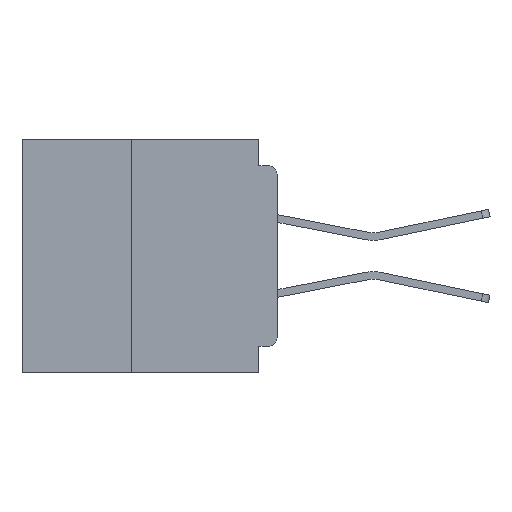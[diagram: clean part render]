
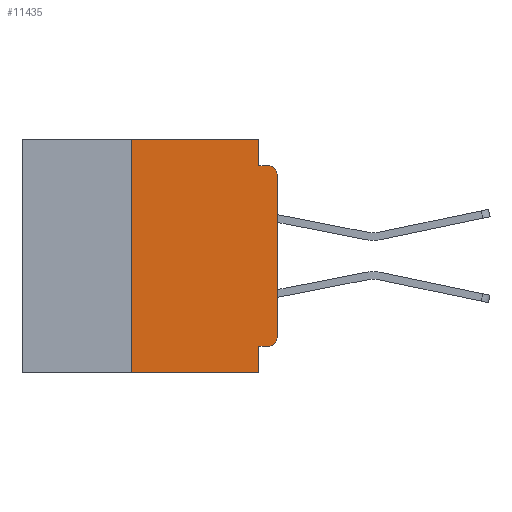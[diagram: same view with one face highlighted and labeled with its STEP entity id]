
A CAD part, left-side view. The second image highlights one B-rep face of the part: STEP entity #11435.
In plain terms, the highlighted planar face has unit normal (-1, 0, 0).
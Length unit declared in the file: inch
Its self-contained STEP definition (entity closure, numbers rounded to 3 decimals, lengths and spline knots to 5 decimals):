
#1499 = CARTESIAN_POINT ( 'NONE',  ( 0., 0.015, -0.34 ) ) ;
#1904 = CARTESIAN_POINT ( 'NONE',  ( 0., 0.437, 0. ) ) ;
#1909 = DIRECTION ( 'NONE',  ( 0., 0., -1. ) ) ;
#2004 = AXIS2_PLACEMENT_3D ( 'NONE', #1904, #37507, #13945 ) ;
#3183 = EDGE_CURVE ( 'NONE', #51028, #47397, #34733, .T. ) ;
#3277 = CARTESIAN_POINT ( 'NONE',  ( 0., 0., -0.34 ) ) ;
#4523 = DIRECTION ( 'NONE',  ( 0., -1., 0. ) ) ;
#4692 = EDGE_CURVE ( 'NONE', #48364, #48477, #16767, .T. ) ;
#5548 = DIRECTION ( 'NONE',  ( 0., 0., -1. ) ) ;
#5969 = PLANE ( 'NONE',  #2004 ) ;
#6402 = CARTESIAN_POINT ( 'NONE',  ( 0., 0.437, -0.4 ) ) ;
#7161 = VECTOR ( 'NONE', #17415, 39.37008 ) ;
#11061 = CARTESIAN_POINT ( 'NONE',  ( 0., 0.015, -0.355 ) ) ;
#11435 = ADVANCED_FACE ( 'NONE', ( #44710 ), #5969, .F. ) ;
#11974 = CARTESIAN_POINT ( 'NONE',  ( 0., 0.015, -0.045 ) ) ;
#12048 = LINE ( 'NONE', #24384, #31739 ) ;
#13144 = VECTOR ( 'NONE', #22391, 39.37008 ) ;
#13276 = EDGE_CURVE ( 'NONE', #36520, #27452, #48739, .T. ) ;
#13356 = CARTESIAN_POINT ( 'NONE',  ( 0., 0.25, -0.4 ) ) ;
#13407 = CARTESIAN_POINT ( 'NONE',  ( 0., 0.031, 0. ) ) ;
#13799 = VECTOR ( 'NONE', #4523, 39.37008 ) ;
#13945 = DIRECTION ( 'NONE',  ( 0., 0., -1. ) ) ;
#16567 = DIRECTION ( 'NONE',  ( 0., 0., 1. ) ) ;
#16674 = LINE ( 'NONE', #45634, #27164 ) ;
#16767 = LINE ( 'NONE', #49928, #28482 ) ;
#16932 = ORIENTED_EDGE ( 'NONE', *, *, #18088, .F. ) ;
#17415 = DIRECTION ( 'NONE',  ( 0., 0., -1. ) ) ;
#18088 = EDGE_CURVE ( 'NONE', #18150, #39817, #40939, .T. ) ;
#18150 = VERTEX_POINT ( 'NONE', #22491 ) ;
#18164 = DIRECTION ( 'NONE',  ( 0., 0., -1. ) ) ;
#18279 = DIRECTION ( 'NONE',  ( 0., 0., 1. ) ) ;
#19345 = EDGE_CURVE ( 'NONE', #31237, #39817, #23690, .T. ) ;
#19841 = ORIENTED_EDGE ( 'NONE', *, *, #19345, .T. ) ;
#20534 = CARTESIAN_POINT ( 'NONE',  ( 0., 0., -0.045 ) ) ;
#20751 = EDGE_CURVE ( 'NONE', #21086, #47397, #38192, .T. ) ;
#21086 = VERTEX_POINT ( 'NONE', #23651 ) ;
#22391 = DIRECTION ( 'NONE',  ( 0., -1., 0. ) ) ;
#22491 = CARTESIAN_POINT ( 'NONE',  ( 0., 0.031, -0.355 ) ) ;
#23246 = ORIENTED_EDGE ( 'NONE', *, *, #38151, .F. ) ;
#23651 = CARTESIAN_POINT ( 'NONE',  ( 0., 0., -0.06 ) ) ;
#23690 = LINE ( 'NONE', #6402, #13144 ) ;
#24384 = CARTESIAN_POINT ( 'NONE',  ( 0., 0., -0.355 ) ) ;
#24808 = CARTESIAN_POINT ( 'NONE',  ( 0., 0.031, -0.045 ) ) ;
#25712 = DIRECTION ( 'NONE',  ( -1., 0., 0. ) ) ;
#26565 = DIRECTION ( 'NONE',  ( 0., -1., 0. ) ) ;
#26682 = CARTESIAN_POINT ( 'NONE',  ( 0., 0.031, 0. ) ) ;
#27164 = VECTOR ( 'NONE', #18279, 39.37008 ) ;
#27452 = VERTEX_POINT ( 'NONE', #3277 ) ;
#27497 = ORIENTED_EDGE ( 'NONE', *, *, #30720, .T. ) ;
#28332 = DIRECTION ( 'NONE',  ( 0., 1., 0. ) ) ;
#28482 = VECTOR ( 'NONE', #26565, 39.37008 ) ;
#29255 = DIRECTION ( 'NONE',  ( -1., 0., 0. ) ) ;
#29857 = CARTESIAN_POINT ( 'NONE',  ( 0., 0.031, -0.4 ) ) ;
#30720 = EDGE_CURVE ( 'NONE', #27452, #21086, #16674, .T. ) ;
#31237 = VERTEX_POINT ( 'NONE', #13356 ) ;
#31739 = VECTOR ( 'NONE', #28332, 39.37008 ) ;
#33677 = CARTESIAN_POINT ( 'NONE',  ( 0., 0.25, 0. ) ) ;
#33735 = ORIENTED_EDGE ( 'NONE', *, *, #36928, .F. ) ;
#34363 = LINE ( 'NONE', #47857, #43547 ) ;
#34733 = LINE ( 'NONE', #20534, #13799 ) ;
#34928 = ORIENTED_EDGE ( 'NONE', *, *, #4692, .F. ) ;
#36520 = VERTEX_POINT ( 'NONE', #11061 ) ;
#36784 = AXIS2_PLACEMENT_3D ( 'NONE', #49075, #25712, #1909 ) ;
#36928 = EDGE_CURVE ( 'NONE', #48477, #51028, #38594, .T. ) ;
#37052 = ORIENTED_EDGE ( 'NONE', *, *, #13276, .T. ) ;
#37507 = DIRECTION ( 'NONE',  ( 1., 0., 0. ) ) ;
#38151 = EDGE_CURVE ( 'NONE', #36520, #18150, #12048, .T. ) ;
#38192 = CIRCLE ( 'NONE', #36784, 0.015 ) ;
#38594 = LINE ( 'NONE', #13407, #7161 ) ;
#39109 = CARTESIAN_POINT ( 'NONE',  ( 0., 0.031, -0.4 ) ) ;
#39721 = VECTOR ( 'NONE', #18164, 39.37008 ) ;
#39817 = VERTEX_POINT ( 'NONE', #39109 ) ;
#40162 = AXIS2_PLACEMENT_3D ( 'NONE', #1499, #29255, #5548 ) ;
#40939 = LINE ( 'NONE', #29857, #39721 ) ;
#43547 = VECTOR ( 'NONE', #16567, 39.37008 ) ;
#43813 = ORIENTED_EDGE ( 'NONE', *, *, #48094, .F. ) ;
#44710 = FACE_OUTER_BOUND ( 'NONE', #49378, .T. ) ;
#45634 = CARTESIAN_POINT ( 'NONE',  ( 0., 0., 0. ) ) ;
#47397 = VERTEX_POINT ( 'NONE', #11974 ) ;
#47857 = CARTESIAN_POINT ( 'NONE',  ( 0., 0.25, -0.4 ) ) ;
#48094 = EDGE_CURVE ( 'NONE', #31237, #48364, #34363, .T. ) ;
#48364 = VERTEX_POINT ( 'NONE', #33677 ) ;
#48477 = VERTEX_POINT ( 'NONE', #26682 ) ;
#48739 = CIRCLE ( 'NONE', #40162, 0.015 ) ;
#49075 = CARTESIAN_POINT ( 'NONE',  ( 0., 0.015, -0.06 ) ) ;
#49378 = EDGE_LOOP ( 'NONE', ( #27497, #49506, #50803, #33735, #34928, #43813, #19841, #16932, #23246, #37052 ) ) ;
#49506 = ORIENTED_EDGE ( 'NONE', *, *, #20751, .T. ) ;
#49928 = CARTESIAN_POINT ( 'NONE',  ( 0., 0.437, 0. ) ) ;
#50803 = ORIENTED_EDGE ( 'NONE', *, *, #3183, .F. ) ;
#51028 = VERTEX_POINT ( 'NONE', #24808 ) ;
